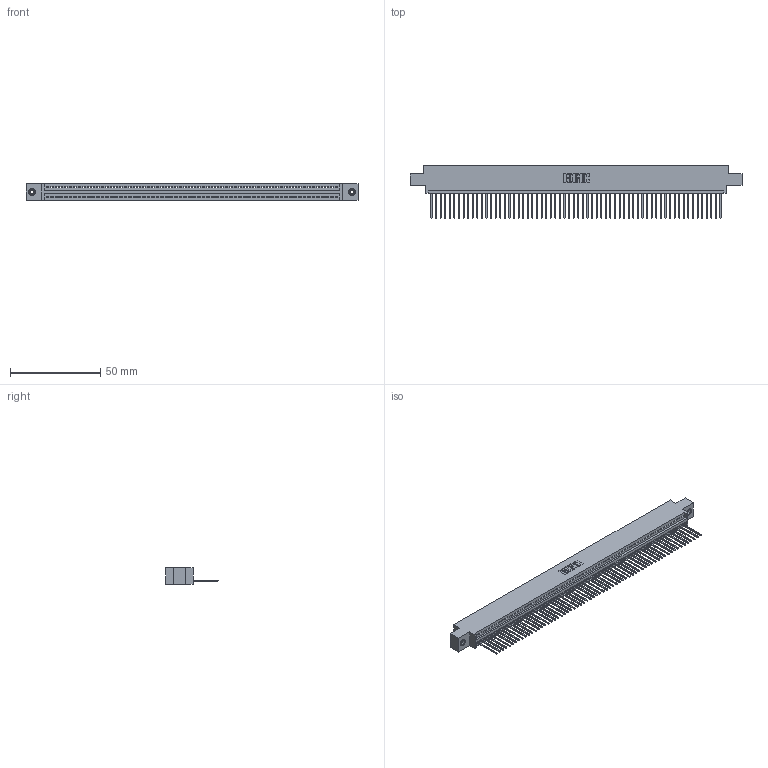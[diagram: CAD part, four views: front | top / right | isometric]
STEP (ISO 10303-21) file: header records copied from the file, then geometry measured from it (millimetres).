
FILE_DESCRIPTION (( 'STEP AP203' ), '1' );
FILE_NAME ('395-064-540-608.STEP', '2019-10-25T02:12:09', ( '' ), ( '' ), 'SwSTEP 2.0', 'SolidWorks 2016', '' );
FILE_SCHEMA (( 'CONFIG_CONTROL_DESIGN' ));
Length unit declared in the file: inch
Products named in the file (4): 345-250-001_345-250-003-102; 345 Part_0.170 Offset - 0.156 Dia-TI; 345-292-001_345-293-140; 395-064-540-608
Assembly tree (67 placements, depth 2):
  395-064-540-608
    345 Part_0.170 Offset - 0.156 Dia-TI
    345-292-001_345-293-140  x64
    345-250-001_345-250-003-102  x2
Bounding box: 183.77 x 29.13 x 9.4 mm (x, y, z)
Volume: 17601.6 mm3; surface area: 24459.2 mm2
Topology: 67 solids, 67 shells, 3902 faces, 11753 edges, 7742 vertices
Faces by surface type: plane 2676, cylinder 1210, cone 12, torus 4
Entity records: 46542 total; most frequent: CARTESIAN_POINT 8043, ORIENTED_EDGE 8034, DIRECTION 7019, EDGE_CURVE 4017, VECTOR 3609, LINE 3609, VERTEX_POINT 2672, AXIS2_PLACEMENT_3D 1705
